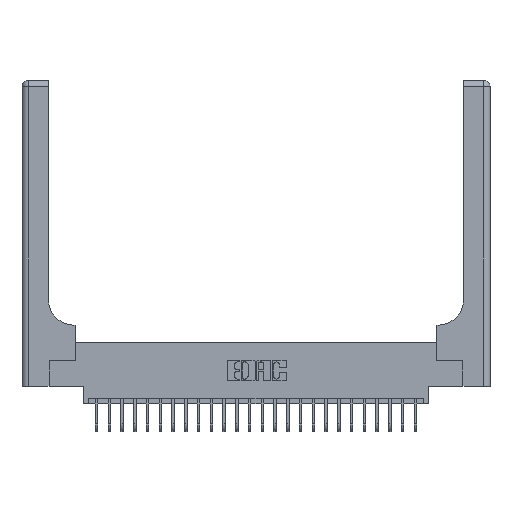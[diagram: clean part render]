
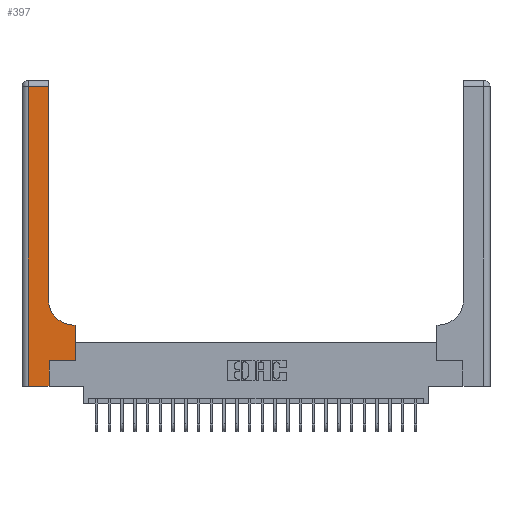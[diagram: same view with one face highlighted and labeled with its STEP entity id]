
A CAD part, top view. The second image highlights one B-rep face of the part: STEP entity #397.
In plain terms, the highlighted planar face has unit normal (0, 0, 1).
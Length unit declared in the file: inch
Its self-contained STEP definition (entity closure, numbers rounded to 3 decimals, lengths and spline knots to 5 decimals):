
#64 = EDGE_CURVE ( 'NONE', #22084, #9860, #22007, .T. ) ;
#397 = ADVANCED_FACE ( 'NONE', ( #4257 ), #25339, .F. ) ;
#777 = DIRECTION ( 'NONE',  ( -1., 0., 0. ) ) ;
#804 = VERTEX_POINT ( 'NONE', #8432 ) ;
#855 = DIRECTION ( 'NONE',  ( 0., 1., 0. ) ) ;
#1275 = VERTEX_POINT ( 'NONE', #20945 ) ;
#1873 = LINE ( 'NONE', #11149, #4403 ) ;
#2393 = DIRECTION ( 'NONE',  ( 1., 0., 0. ) ) ;
#2397 = ORIENTED_EDGE ( 'NONE', *, *, #15655, .T. ) ;
#3070 = DIRECTION ( 'NONE',  ( 0., -1., 0. ) ) ;
#3965 = CARTESIAN_POINT ( 'NONE',  ( 0.26, 0.6, 0.37 ) ) ;
#4257 = FACE_OUTER_BOUND ( 'NONE', #8652, .T. ) ;
#4315 = CARTESIAN_POINT ( 'NONE',  ( 0.528, 0.25, 0.37 ) ) ;
#4403 = VECTOR ( 'NONE', #12370, 39.37008 ) ;
#4648 = ORIENTED_EDGE ( 'NONE', *, *, #9474, .T. ) ;
#5002 = CARTESIAN_POINT ( 'NONE',  ( 0.528, 0.6, 0.37 ) ) ;
#5149 = CARTESIAN_POINT ( 'NONE',  ( 0., 3., 0.37 ) ) ;
#5444 = ORIENTED_EDGE ( 'NONE', *, *, #6300, .T. ) ;
#5604 = VECTOR ( 'NONE', #777, 39.37008 ) ;
#5911 = CARTESIAN_POINT ( 'NONE',  ( 0.06, 0., 0.37 ) ) ;
#6274 = VERTEX_POINT ( 'NONE', #16524 ) ;
#6279 = VERTEX_POINT ( 'NONE', #24687 ) ;
#6300 = EDGE_CURVE ( 'NONE', #1275, #10389, #20981, .T. ) ;
#6408 = ORIENTED_EDGE ( 'NONE', *, *, #9207, .T. ) ;
#7106 = AXIS2_PLACEMENT_3D ( 'NONE', #24909, #25270, #13127 ) ;
#7555 = VECTOR ( 'NONE', #2393, 39.37008 ) ;
#7680 = VECTOR ( 'NONE', #855, 39.37008 ) ;
#7888 = DIRECTION ( 'NONE',  ( -1., 0., 0. ) ) ;
#7894 = ORIENTED_EDGE ( 'NONE', *, *, #8753, .T. ) ;
#8167 = EDGE_CURVE ( 'NONE', #804, #6274, #1873, .T. ) ;
#8173 = VECTOR ( 'NONE', #7888, 39.37008 ) ;
#8432 = CARTESIAN_POINT ( 'NONE',  ( 0.26, 0.85, 0.37 ) ) ;
#8606 = AXIS2_PLACEMENT_3D ( 'NONE', #5149, #9260, #15147 ) ;
#8652 = EDGE_LOOP ( 'NONE', ( #24010, #18959, #21422, #4648, #2397, #7894, #5444, #6408, #11403 ) ) ;
#8753 = EDGE_CURVE ( 'NONE', #13235, #1275, #14199, .T. ) ;
#9160 = CARTESIAN_POINT ( 'NONE',  ( 0.06, 3., 0.37 ) ) ;
#9207 = EDGE_CURVE ( 'NONE', #10389, #19441, #23668, .T. ) ;
#9260 = DIRECTION ( 'NONE',  ( 0., 0., -1. ) ) ;
#9444 = VECTOR ( 'NONE', #14869, 39.37008 ) ;
#9474 = EDGE_CURVE ( 'NONE', #9860, #6279, #24608, .T. ) ;
#9860 = VERTEX_POINT ( 'NONE', #5911 ) ;
#10389 = VERTEX_POINT ( 'NONE', #5002 ) ;
#11149 = CARTESIAN_POINT ( 'NONE',  ( 0.26, 3., 0.37 ) ) ;
#11403 = ORIENTED_EDGE ( 'NONE', *, *, #21480, .T. ) ;
#11466 = DIRECTION ( 'NONE',  ( 0., 1., 0. ) ) ;
#12370 = DIRECTION ( 'NONE',  ( 0., 1., 0. ) ) ;
#12846 = VECTOR ( 'NONE', #11466, 39.37008 ) ;
#13127 = DIRECTION ( 'NONE',  ( 1., 0., 0. ) ) ;
#13235 = VERTEX_POINT ( 'NONE', #22123 ) ;
#14199 = LINE ( 'NONE', #18879, #7555 ) ;
#14869 = DIRECTION ( 'NONE',  ( 1., 0., 0. ) ) ;
#15147 = DIRECTION ( 'NONE',  ( -1., 0., 0. ) ) ;
#15655 = EDGE_CURVE ( 'NONE', #6279, #13235, #24237, .T. ) ;
#16524 = CARTESIAN_POINT ( 'NONE',  ( 0.26, 2.94, 0.37 ) ) ;
#16608 = CARTESIAN_POINT ( 'NONE',  ( 0., 0., 0.37 ) ) ;
#18879 = CARTESIAN_POINT ( 'NONE',  ( 0.265, 0.25, 0.37 ) ) ;
#18959 = ORIENTED_EDGE ( 'NONE', *, *, #22211, .T. ) ;
#19441 = VERTEX_POINT ( 'NONE', #26249 ) ;
#20945 = CARTESIAN_POINT ( 'NONE',  ( 0.528, 0.25, 0.37 ) ) ;
#20981 = LINE ( 'NONE', #4315, #7680 ) ;
#21422 = ORIENTED_EDGE ( 'NONE', *, *, #64, .T. ) ;
#21480 = EDGE_CURVE ( 'NONE', #19441, #804, #22368, .T. ) ;
#21716 = VECTOR ( 'NONE', #3070, 39.37008 ) ;
#22007 = LINE ( 'NONE', #9160, #21716 ) ;
#22084 = VERTEX_POINT ( 'NONE', #22651 ) ;
#22123 = CARTESIAN_POINT ( 'NONE',  ( 0.265, 0.25, 0.37 ) ) ;
#22211 = EDGE_CURVE ( 'NONE', #6274, #22084, #24594, .T. ) ;
#22368 = CIRCLE ( 'NONE', #7106, 0.25 ) ;
#22651 = CARTESIAN_POINT ( 'NONE',  ( 0.06, 2.94, 0.37 ) ) ;
#23668 = LINE ( 'NONE', #3965, #8173 ) ;
#24010 = ORIENTED_EDGE ( 'NONE', *, *, #8167, .T. ) ;
#24237 = LINE ( 'NONE', #26221, #12846 ) ;
#24594 = LINE ( 'NONE', #25066, #5604 ) ;
#24608 = LINE ( 'NONE', #16608, #9444 ) ;
#24687 = CARTESIAN_POINT ( 'NONE',  ( 0.265, 0., 0.37 ) ) ;
#24909 = CARTESIAN_POINT ( 'NONE',  ( 0.51, 0.85, 0.37 ) ) ;
#25066 = CARTESIAN_POINT ( 'NONE',  ( 0., 2.94, 0.37 ) ) ;
#25270 = DIRECTION ( 'NONE',  ( 0., 0., -1. ) ) ;
#25339 = PLANE ( 'NONE',  #8606 ) ;
#26221 = CARTESIAN_POINT ( 'NONE',  ( 0.265, 0., 0.37 ) ) ;
#26249 = CARTESIAN_POINT ( 'NONE',  ( 0.51, 0.6, 0.37 ) ) ;
